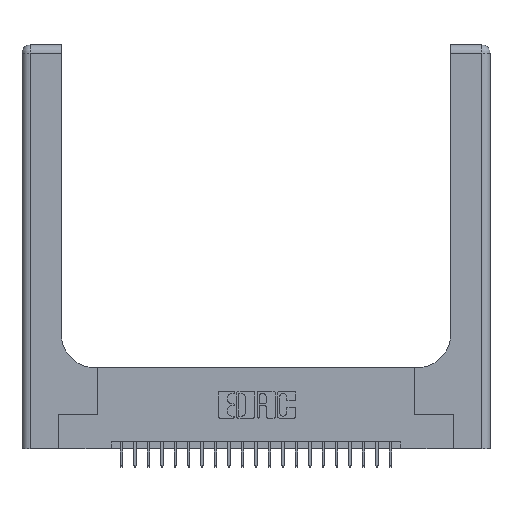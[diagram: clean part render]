
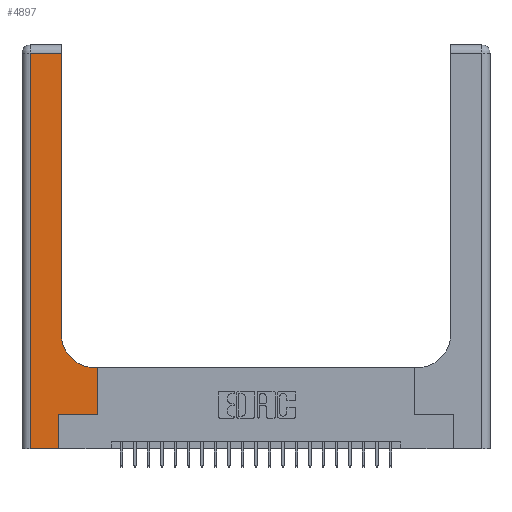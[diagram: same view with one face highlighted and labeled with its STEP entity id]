
A CAD part, top view. The second image highlights one B-rep face of the part: STEP entity #4897.
In plain terms, the highlighted planar face has unit normal (0, 0, 1).
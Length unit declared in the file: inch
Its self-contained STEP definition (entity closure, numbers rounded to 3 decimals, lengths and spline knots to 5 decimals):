
#378 = DIRECTION ( 'NONE',  ( 0., 1., 0. ) ) ;
#717 = DIRECTION ( 'NONE',  ( 1., 0., 0. ) ) ;
#739 = CARTESIAN_POINT ( 'NONE',  ( 0.5585, 0.25, 0.37 ) ) ;
#1039 = CARTESIAN_POINT ( 'NONE',  ( 0.2915, 3., 0.37 ) ) ;
#1175 = VERTEX_POINT ( 'NONE', #24024 ) ;
#1244 = VERTEX_POINT ( 'NONE', #7828 ) ;
#1363 = DIRECTION ( 'NONE',  ( 0., 0., -1. ) ) ;
#2490 = CARTESIAN_POINT ( 'NONE',  ( 0.269, 0., 0.37 ) ) ;
#2576 = LINE ( 'NONE', #12037, #4124 ) ;
#2642 = CARTESIAN_POINT ( 'NONE',  ( 0.06, 3., 0.37 ) ) ;
#2893 = ORIENTED_EDGE ( 'NONE', *, *, #20820, .T. ) ;
#3153 = CARTESIAN_POINT ( 'NONE',  ( 0.269, 0.25, 0.37 ) ) ;
#3334 = CARTESIAN_POINT ( 'NONE',  ( 0.06, 2.94, 0.37 ) ) ;
#3438 = ORIENTED_EDGE ( 'NONE', *, *, #13277, .T. ) ;
#3862 = VECTOR ( 'NONE', #12604, 39.37008 ) ;
#4017 = DIRECTION ( 'NONE',  ( 1., 0., 0. ) ) ;
#4124 = VECTOR ( 'NONE', #9791, 39.37008 ) ;
#4332 = ORIENTED_EDGE ( 'NONE', *, *, #20511, .T. ) ;
#4864 = VERTEX_POINT ( 'NONE', #3334 ) ;
#4897 = ADVANCED_FACE ( 'NONE', ( #14426 ), #20289, .F. ) ;
#5349 = VECTOR ( 'NONE', #20529, 39.37008 ) ;
#5587 = CIRCLE ( 'NONE', #14717, 0.25 ) ;
#6251 = ORIENTED_EDGE ( 'NONE', *, *, #14397, .T. ) ;
#7402 = VECTOR ( 'NONE', #11931, 39.37008 ) ;
#7437 = EDGE_CURVE ( 'NONE', #16052, #1244, #15276, .T. ) ;
#7661 = AXIS2_PLACEMENT_3D ( 'NONE', #18417, #1363, #8953 ) ;
#7828 = CARTESIAN_POINT ( 'NONE',  ( 0.5585, 0.6, 0.37 ) ) ;
#8918 = CARTESIAN_POINT ( 'NONE',  ( 0.269, 0., 0.37 ) ) ;
#8953 = DIRECTION ( 'NONE',  ( -1., 0., 0. ) ) ;
#8980 = VERTEX_POINT ( 'NONE', #8918 ) ;
#9791 = DIRECTION ( 'NONE',  ( -1., 0., 0. ) ) ;
#10450 = DIRECTION ( 'NONE',  ( -1., 0., 0. ) ) ;
#11030 = EDGE_CURVE ( 'NONE', #13276, #14080, #22098, .T. ) ;
#11134 = VECTOR ( 'NONE', #717, 39.37008 ) ;
#11796 = CARTESIAN_POINT ( 'NONE',  ( 0., 0., 0.37 ) ) ;
#11931 = DIRECTION ( 'NONE',  ( 0., 1., 0. ) ) ;
#12037 = CARTESIAN_POINT ( 'NONE',  ( 0., 2.94, 0.37 ) ) ;
#12064 = LINE ( 'NONE', #2490, #18393 ) ;
#12604 = DIRECTION ( 'NONE',  ( 0., 1., 0. ) ) ;
#12625 = CARTESIAN_POINT ( 'NONE',  ( 0.2915, 0.85, 0.37 ) ) ;
#12915 = LINE ( 'NONE', #11796, #11134 ) ;
#13276 = VERTEX_POINT ( 'NONE', #12625 ) ;
#13277 = EDGE_CURVE ( 'NONE', #1175, #16052, #20210, .T. ) ;
#13678 = VERTEX_POINT ( 'NONE', #15066 ) ;
#13706 = ORIENTED_EDGE ( 'NONE', *, *, #11030, .T. ) ;
#14080 = VERTEX_POINT ( 'NONE', #17741 ) ;
#14397 = EDGE_CURVE ( 'NONE', #13678, #13276, #5587, .T. ) ;
#14426 = FACE_OUTER_BOUND ( 'NONE', #24546, .T. ) ;
#14717 = AXIS2_PLACEMENT_3D ( 'NONE', #20843, #15709, #4017 ) ;
#15066 = CARTESIAN_POINT ( 'NONE',  ( 0.5415, 0.6, 0.37 ) ) ;
#15276 = LINE ( 'NONE', #17170, #7402 ) ;
#15686 = EDGE_CURVE ( 'NONE', #16855, #8980, #12915, .T. ) ;
#15709 = DIRECTION ( 'NONE',  ( 0., 0., -1. ) ) ;
#16052 = VERTEX_POINT ( 'NONE', #739 ) ;
#16854 = DIRECTION ( 'NONE',  ( 1., 0., 0. ) ) ;
#16855 = VERTEX_POINT ( 'NONE', #19767 ) ;
#17170 = CARTESIAN_POINT ( 'NONE',  ( 0.5585, 0.25, 0.37 ) ) ;
#17741 = CARTESIAN_POINT ( 'NONE',  ( 0.2915, 2.94, 0.37 ) ) ;
#17915 = CARTESIAN_POINT ( 'NONE',  ( 0.2915, 0.6, 0.37 ) ) ;
#18393 = VECTOR ( 'NONE', #378, 39.37008 ) ;
#18417 = CARTESIAN_POINT ( 'NONE',  ( 0., 3., 0.37 ) ) ;
#19024 = EDGE_CURVE ( 'NONE', #8980, #1175, #12064, .T. ) ;
#19229 = VECTOR ( 'NONE', #10450, 39.37008 ) ;
#19767 = CARTESIAN_POINT ( 'NONE',  ( 0.06, 0., 0.37 ) ) ;
#20009 = ORIENTED_EDGE ( 'NONE', *, *, #19024, .T. ) ;
#20210 = LINE ( 'NONE', #3153, #22651 ) ;
#20286 = LINE ( 'NONE', #2642, #5349 ) ;
#20289 = PLANE ( 'NONE',  #7661 ) ;
#20511 = EDGE_CURVE ( 'NONE', #1244, #13678, #22292, .T. ) ;
#20529 = DIRECTION ( 'NONE',  ( 0., -1., 0. ) ) ;
#20820 = EDGE_CURVE ( 'NONE', #14080, #4864, #2576, .T. ) ;
#20843 = CARTESIAN_POINT ( 'NONE',  ( 0.5415, 0.85, 0.37 ) ) ;
#21300 = ORIENTED_EDGE ( 'NONE', *, *, #7437, .T. ) ;
#21644 = EDGE_CURVE ( 'NONE', #4864, #16855, #20286, .T. ) ;
#22098 = LINE ( 'NONE', #1039, #3862 ) ;
#22292 = LINE ( 'NONE', #17915, #19229 ) ;
#22651 = VECTOR ( 'NONE', #16854, 39.37008 ) ;
#22837 = ORIENTED_EDGE ( 'NONE', *, *, #15686, .T. ) ;
#24024 = CARTESIAN_POINT ( 'NONE',  ( 0.269, 0.25, 0.37 ) ) ;
#24057 = ORIENTED_EDGE ( 'NONE', *, *, #21644, .T. ) ;
#24546 = EDGE_LOOP ( 'NONE', ( #13706, #2893, #24057, #22837, #20009, #3438, #21300, #4332, #6251 ) ) ;
